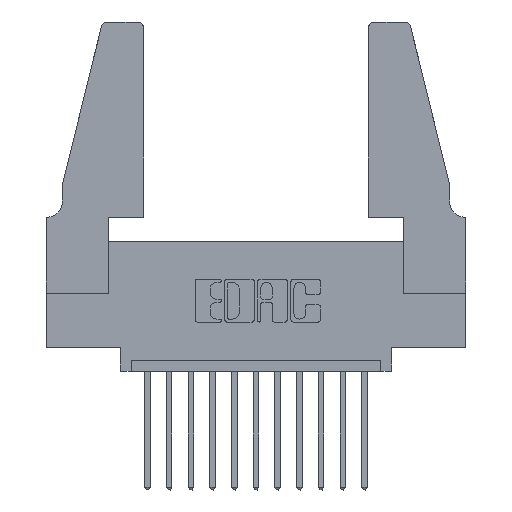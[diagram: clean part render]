
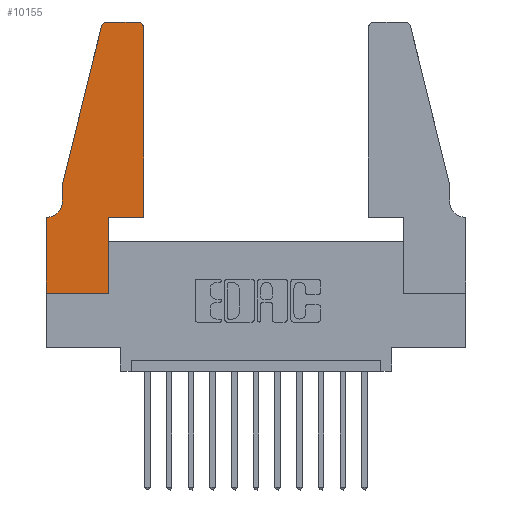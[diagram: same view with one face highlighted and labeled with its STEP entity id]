
A CAD part, top view. The second image highlights one B-rep face of the part: STEP entity #10155.
In plain terms, the highlighted planar face has unit normal (0, 0, 1).
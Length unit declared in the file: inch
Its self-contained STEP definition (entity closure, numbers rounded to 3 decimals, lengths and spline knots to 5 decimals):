
#47 = EDGE_CURVE ( 'NONE', #975, #11227, #1218, .T. ) ;
#442 = VECTOR ( 'NONE', #7570, 39.37008 ) ;
#481 = VECTOR ( 'NONE', #12152, 39.37008 ) ;
#525 = DIRECTION ( 'NONE',  ( 0., -1., 0. ) ) ;
#556 = CARTESIAN_POINT ( 'NONE',  ( 0.0755, 0.5, 0.37 ) ) ;
#738 = PLANE ( 'NONE',  #12643 ) ;
#788 = DIRECTION ( 'NONE',  ( 1., 0., 0. ) ) ;
#899 = CARTESIAN_POINT ( 'NONE',  ( 0.4505, 1.22, 0.37 ) ) ;
#950 = LINE ( 'NONE', #2303, #13631 ) ;
#958 = CARTESIAN_POINT ( 'NONE',  ( 0., 0., 0.37 ) ) ;
#975 = VERTEX_POINT ( 'NONE', #4504 ) ;
#998 = DIRECTION ( 'NONE',  ( 1., 0., 0. ) ) ;
#1070 = DIRECTION ( 'NONE',  ( 1., 0., 0. ) ) ;
#1218 = LINE ( 'NONE', #10559, #13534 ) ;
#1484 = CARTESIAN_POINT ( 'NONE',  ( 0.2865, 0., 0.37 ) ) ;
#1566 = CARTESIAN_POINT ( 'NONE',  ( 0.0755, 0.5, 0.37 ) ) ;
#2051 = EDGE_CURVE ( 'NONE', #11311, #975, #7432, .T. ) ;
#2300 = ORIENTED_EDGE ( 'NONE', *, *, #5266, .T. ) ;
#2303 = CARTESIAN_POINT ( 'NONE',  ( 0.0755, 0.5, 0.37 ) ) ;
#2308 = EDGE_CURVE ( 'NONE', #14249, #8576, #7966, .T. ) ;
#2446 = CARTESIAN_POINT ( 'NONE',  ( 0.0755, 0.42, 0.37 ) ) ;
#2452 = VERTEX_POINT ( 'NONE', #6365 ) ;
#3012 = CARTESIAN_POINT ( 'NONE',  ( 0., 0.35, 0.37 ) ) ;
#3118 = DIRECTION ( 'NONE',  ( 0., 0., -1. ) ) ;
#3251 = VERTEX_POINT ( 'NONE', #9726 ) ;
#3832 = VERTEX_POINT ( 'NONE', #899 ) ;
#4165 = CARTESIAN_POINT ( 'NONE',  ( 0.2865, 0.35, 0.37 ) ) ;
#4373 = ORIENTED_EDGE ( 'NONE', *, *, #8718, .T. ) ;
#4415 = LINE ( 'NONE', #8465, #13138 ) ;
#4504 = CARTESIAN_POINT ( 'NONE',  ( 0.0055, 0.35, 0.37 ) ) ;
#4639 = CARTESIAN_POINT ( 'NONE',  ( 0.25487, 1.22718, 0.37 ) ) ;
#4918 = VECTOR ( 'NONE', #7030, 39.37008 ) ;
#5064 = AXIS2_PLACEMENT_3D ( 'NONE', #6483, #3118, #7771 ) ;
#5139 = ORIENTED_EDGE ( 'NONE', *, *, #11793, .T. ) ;
#5266 = EDGE_CURVE ( 'NONE', #8734, #3251, #14218, .T. ) ;
#5900 = ORIENTED_EDGE ( 'NONE', *, *, #12700, .T. ) ;
#6025 = DIRECTION ( 'NONE',  ( -1., 0., 0. ) ) ;
#6365 = CARTESIAN_POINT ( 'NONE',  ( 0., 0., 0.37 ) ) ;
#6417 = EDGE_CURVE ( 'NONE', #3251, #14681, #10044, .T. ) ;
#6483 = CARTESIAN_POINT ( 'NONE',  ( 0.0055, 0.42, 0.37 ) ) ;
#6491 = DIRECTION ( 'NONE',  ( 1., 0., 0. ) ) ;
#6498 = ORIENTED_EDGE ( 'NONE', *, *, #11625, .T. ) ;
#6648 = EDGE_LOOP ( 'NONE', ( #2300, #7332, #14172, #4373, #8423, #12931, #6498, #6948, #5139, #13543, #13470, #5900 ) ) ;
#6707 = CARTESIAN_POINT ( 'NONE',  ( 0.4505, 0.35, 0.37 ) ) ;
#6766 = AXIS2_PLACEMENT_3D ( 'NONE', #7929, #11382, #1070 ) ;
#6948 = ORIENTED_EDGE ( 'NONE', *, *, #14116, .T. ) ;
#7030 = DIRECTION ( 'NONE',  ( 1., 0., 0. ) ) ;
#7063 = AXIS2_PLACEMENT_3D ( 'NONE', #12358, #7636, #6491 ) ;
#7312 = CARTESIAN_POINT ( 'NONE',  ( 0.4205, 1.25, 0.37 ) ) ;
#7332 = ORIENTED_EDGE ( 'NONE', *, *, #6417, .T. ) ;
#7432 = CIRCLE ( 'NONE', #5064, 0.07 ) ;
#7570 = DIRECTION ( 'NONE',  ( 0., 1., 0. ) ) ;
#7636 = DIRECTION ( 'NONE',  ( 0., 0., 1. ) ) ;
#7771 = DIRECTION ( 'NONE',  ( -1., 0., 0. ) ) ;
#7929 = CARTESIAN_POINT ( 'NONE',  ( 0.4205, 1.22, 0.37 ) ) ;
#7966 = LINE ( 'NONE', #14010, #4918 ) ;
#8423 = ORIENTED_EDGE ( 'NONE', *, *, #2051, .T. ) ;
#8465 = CARTESIAN_POINT ( 'NONE',  ( 0., 0., 0.37 ) ) ;
#8576 = VERTEX_POINT ( 'NONE', #6707 ) ;
#8718 = EDGE_CURVE ( 'NONE', #10084, #11311, #9498, .T. ) ;
#8734 = VERTEX_POINT ( 'NONE', #7312 ) ;
#8812 = VECTOR ( 'NONE', #998, 39.37008 ) ;
#8836 = CARTESIAN_POINT ( 'NONE',  ( 0.4505, 0.35, 0.37 ) ) ;
#8937 = VERTEX_POINT ( 'NONE', #1484 ) ;
#9288 = FACE_OUTER_BOUND ( 'NONE', #6648, .T. ) ;
#9498 = LINE ( 'NONE', #1566, #10216 ) ;
#9726 = CARTESIAN_POINT ( 'NONE',  ( 0.284, 1.25, 0.37 ) ) ;
#10044 = CIRCLE ( 'NONE', #7063, 0.03 ) ;
#10084 = VERTEX_POINT ( 'NONE', #556 ) ;
#10155 = ADVANCED_FACE ( 'NONE', ( #9288 ), #738, .T. ) ;
#10208 = CARTESIAN_POINT ( 'NONE',  ( 0., 0.35, 0.37 ) ) ;
#10216 = VECTOR ( 'NONE', #10752, 39.37008 ) ;
#10439 = CIRCLE ( 'NONE', #6766, 0.03 ) ;
#10559 = CARTESIAN_POINT ( 'NONE',  ( 0.0755, 0.35, 0.37 ) ) ;
#10572 = LINE ( 'NONE', #958, #8812 ) ;
#10752 = DIRECTION ( 'NONE',  ( 0., -1., 0. ) ) ;
#11038 = EDGE_CURVE ( 'NONE', #8576, #3832, #11879, .T. ) ;
#11123 = CARTESIAN_POINT ( 'NONE',  ( 0.2865, 0.35, 0.37 ) ) ;
#11227 = VERTEX_POINT ( 'NONE', #10208 ) ;
#11265 = CARTESIAN_POINT ( 'NONE',  ( 0.2605, 1.25, 0.37 ) ) ;
#11311 = VERTEX_POINT ( 'NONE', #2446 ) ;
#11382 = DIRECTION ( 'NONE',  ( 0., 0., 1. ) ) ;
#11625 = EDGE_CURVE ( 'NONE', #11227, #2452, #4415, .T. ) ;
#11793 = EDGE_CURVE ( 'NONE', #8937, #14249, #12941, .T. ) ;
#11879 = LINE ( 'NONE', #8836, #442 ) ;
#12152 = DIRECTION ( 'NONE',  ( 0., 1., 0. ) ) ;
#12221 = DIRECTION ( 'NONE',  ( 0., 0., 1. ) ) ;
#12358 = CARTESIAN_POINT ( 'NONE',  ( 0.284, 1.22, 0.37 ) ) ;
#12574 = DIRECTION ( 'NONE',  ( -0.239, -0.971, 0. ) ) ;
#12643 = AXIS2_PLACEMENT_3D ( 'NONE', #3012, #12221, #788 ) ;
#12700 = EDGE_CURVE ( 'NONE', #3832, #8734, #10439, .T. ) ;
#12931 = ORIENTED_EDGE ( 'NONE', *, *, #47, .T. ) ;
#12941 = LINE ( 'NONE', #4165, #481 ) ;
#12942 = VECTOR ( 'NONE', #13549, 39.37008 ) ;
#13138 = VECTOR ( 'NONE', #525, 39.37008 ) ;
#13435 = EDGE_CURVE ( 'NONE', #14681, #10084, #950, .T. ) ;
#13470 = ORIENTED_EDGE ( 'NONE', *, *, #11038, .T. ) ;
#13534 = VECTOR ( 'NONE', #6025, 39.37008 ) ;
#13543 = ORIENTED_EDGE ( 'NONE', *, *, #2308, .T. ) ;
#13549 = DIRECTION ( 'NONE',  ( -1., 0., 0. ) ) ;
#13631 = VECTOR ( 'NONE', #12574, 39.37008 ) ;
#14010 = CARTESIAN_POINT ( 'NONE',  ( 0.4505, 0.35, 0.37 ) ) ;
#14116 = EDGE_CURVE ( 'NONE', #2452, #8937, #10572, .T. ) ;
#14172 = ORIENTED_EDGE ( 'NONE', *, *, #13435, .T. ) ;
#14218 = LINE ( 'NONE', #11265, #12942 ) ;
#14249 = VERTEX_POINT ( 'NONE', #11123 ) ;
#14681 = VERTEX_POINT ( 'NONE', #4639 ) ;
